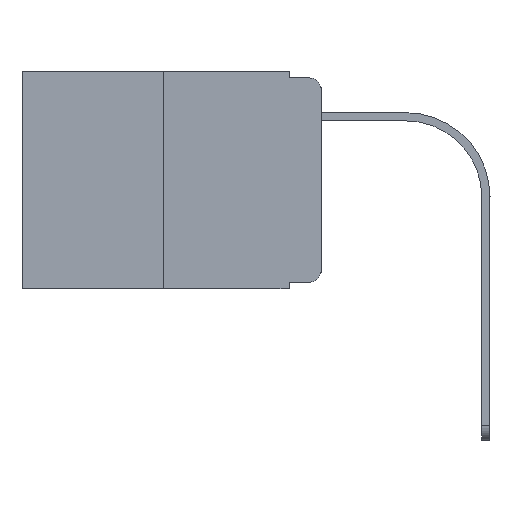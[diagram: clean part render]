
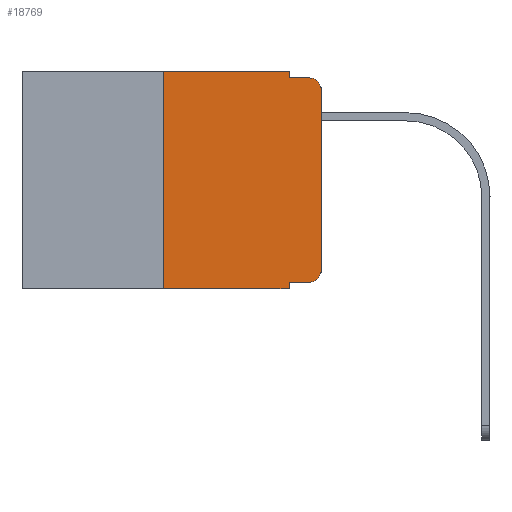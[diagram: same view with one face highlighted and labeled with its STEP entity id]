
A CAD part, left-side view. The second image highlights one B-rep face of the part: STEP entity #18769.
In plain terms, the highlighted planar face has unit normal (-1, 0, 0).
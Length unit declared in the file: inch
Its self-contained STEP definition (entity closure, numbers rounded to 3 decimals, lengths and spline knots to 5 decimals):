
#757 = CARTESIAN_POINT ( 'NONE',  ( 0., 0.051, 0. ) ) ;
#1291 = EDGE_CURVE ( 'NONE', #17932, #7058, #20796, .T. ) ;
#1302 = CARTESIAN_POINT ( 'NONE',  ( 0., 0.02, -0.03 ) ) ;
#1710 = VECTOR ( 'NONE', #16569, 39.37008 ) ;
#1801 = LINE ( 'NONE', #15837, #15571 ) ;
#2091 = LINE ( 'NONE', #12773, #8432 ) ;
#2322 = DIRECTION ( 'NONE',  ( 0., -1., 0. ) ) ;
#2405 = CARTESIAN_POINT ( 'NONE',  ( 0., 0.051, 0. ) ) ;
#2436 = LINE ( 'NONE', #16945, #10281 ) ;
#2755 = VERTEX_POINT ( 'NONE', #18517 ) ;
#2842 = CARTESIAN_POINT ( 'NONE',  ( 0., 0., -0.313 ) ) ;
#3052 = DIRECTION ( 'NONE',  ( 0., 0., -1. ) ) ;
#3207 = DIRECTION ( 'NONE',  ( 0., 0., -1. ) ) ;
#4050 = DIRECTION ( 'NONE',  ( 0., -1., 0. ) ) ;
#4352 = CIRCLE ( 'NONE', #13968, 0.02 ) ;
#4408 = AXIS2_PLACEMENT_3D ( 'NONE', #8864, #19084, #19208 ) ;
#5575 = CARTESIAN_POINT ( 'NONE',  ( 0., 0.051, -0.343 ) ) ;
#5731 = CARTESIAN_POINT ( 'NONE',  ( 0., 0.25, 0. ) ) ;
#5785 = EDGE_CURVE ( 'NONE', #12706, #19299, #18318, .T. ) ;
#6002 = DIRECTION ( 'NONE',  ( 0., 0., 1. ) ) ;
#6439 = VERTEX_POINT ( 'NONE', #5575 ) ;
#6681 = PLANE ( 'NONE',  #4408 ) ;
#7058 = VERTEX_POINT ( 'NONE', #12872 ) ;
#7110 = FACE_OUTER_BOUND ( 'NONE', #17758, .T. ) ;
#7277 = ORIENTED_EDGE ( 'NONE', *, *, #16275, .T. ) ;
#7278 = CARTESIAN_POINT ( 'NONE',  ( 0., 0.473, 0. ) ) ;
#8432 = VECTOR ( 'NONE', #19842, 39.37008 ) ;
#8864 = CARTESIAN_POINT ( 'NONE',  ( 0., 0.473, 0. ) ) ;
#9947 = CARTESIAN_POINT ( 'NONE',  ( 0., 0.02, -0.313 ) ) ;
#10281 = VECTOR ( 'NONE', #2322, 39.37008 ) ;
#10312 = EDGE_CURVE ( 'NONE', #14915, #22020, #2091, .T. ) ;
#10355 = EDGE_CURVE ( 'NONE', #14915, #6439, #2436, .T. ) ;
#10602 = DIRECTION ( 'NONE',  ( 0., 0., -1. ) ) ;
#10775 = ORIENTED_EDGE ( 'NONE', *, *, #10355, .T. ) ;
#11342 = CARTESIAN_POINT ( 'NONE',  ( 0., 0., 0. ) ) ;
#11962 = CARTESIAN_POINT ( 'NONE',  ( 0., 0.051, -0.333 ) ) ;
#11995 = DIRECTION ( 'NONE',  ( 0., -1., 0. ) ) ;
#12545 = EDGE_CURVE ( 'NONE', #17932, #6439, #1801, .T. ) ;
#12706 = VERTEX_POINT ( 'NONE', #757 ) ;
#12773 = CARTESIAN_POINT ( 'NONE',  ( 0., 0.25, 0. ) ) ;
#12872 = CARTESIAN_POINT ( 'NONE',  ( 0., 0.02, -0.333 ) ) ;
#13108 = VERTEX_POINT ( 'NONE', #14766 ) ;
#13968 = AXIS2_PLACEMENT_3D ( 'NONE', #9947, #21066, #3207 ) ;
#14037 = ORIENTED_EDGE ( 'NONE', *, *, #21819, .T. ) ;
#14766 = CARTESIAN_POINT ( 'NONE',  ( 0., 0.02, -0.01 ) ) ;
#14915 = VERTEX_POINT ( 'NONE', #20787 ) ;
#14977 = ORIENTED_EDGE ( 'NONE', *, *, #22851, .F. ) ;
#15316 = ORIENTED_EDGE ( 'NONE', *, *, #21644, .T. ) ;
#15571 = VECTOR ( 'NONE', #10602, 39.37008 ) ;
#15625 = VERTEX_POINT ( 'NONE', #2842 ) ;
#15837 = CARTESIAN_POINT ( 'NONE',  ( 0., 0.051, 0. ) ) ;
#15996 = CARTESIAN_POINT ( 'NONE',  ( 0., 0.051, -0.01 ) ) ;
#16161 = ORIENTED_EDGE ( 'NONE', *, *, #5785, .F. ) ;
#16275 = EDGE_CURVE ( 'NONE', #2755, #13108, #17343, .T. ) ;
#16297 = LINE ( 'NONE', #11342, #19892 ) ;
#16569 = DIRECTION ( 'NONE',  ( 0., 0., -1. ) ) ;
#16658 = ORIENTED_EDGE ( 'NONE', *, *, #10312, .F. ) ;
#16863 = CARTESIAN_POINT ( 'NONE',  ( 0., 0.051, -0.333 ) ) ;
#16945 = CARTESIAN_POINT ( 'NONE',  ( 0., 0.473, -0.343 ) ) ;
#17343 = CIRCLE ( 'NONE', #17709, 0.02 ) ;
#17374 = VECTOR ( 'NONE', #4050, 39.37008 ) ;
#17709 = AXIS2_PLACEMENT_3D ( 'NONE', #1302, #20683, #3052 ) ;
#17758 = EDGE_LOOP ( 'NONE', ( #15316, #7277, #22328, #16161, #14977, #16658, #10775, #22904, #18558, #14037 ) ) ;
#17929 = VECTOR ( 'NONE', #11995, 39.37008 ) ;
#17932 = VERTEX_POINT ( 'NONE', #11962 ) ;
#17958 = EDGE_CURVE ( 'NONE', #19299, #13108, #22823, .T. ) ;
#18318 = LINE ( 'NONE', #2405, #1710 ) ;
#18517 = CARTESIAN_POINT ( 'NONE',  ( 0., 0., -0.03 ) ) ;
#18558 = ORIENTED_EDGE ( 'NONE', *, *, #1291, .T. ) ;
#18769 = ADVANCED_FACE ( 'NONE', ( #7110 ), #6681, .F. ) ;
#19084 = DIRECTION ( 'NONE',  ( 1., 0., 0. ) ) ;
#19208 = DIRECTION ( 'NONE',  ( 0., 0., -1. ) ) ;
#19299 = VERTEX_POINT ( 'NONE', #15996 ) ;
#19362 = DIRECTION ( 'NONE',  ( 0., -1., 0. ) ) ;
#19465 = CARTESIAN_POINT ( 'NONE',  ( 0., 0.051, -0.01 ) ) ;
#19607 = VECTOR ( 'NONE', #19362, 39.37008 ) ;
#19842 = DIRECTION ( 'NONE',  ( 0., 0., 1. ) ) ;
#19892 = VECTOR ( 'NONE', #6002, 39.37008 ) ;
#20683 = DIRECTION ( 'NONE',  ( -1., 0., 0. ) ) ;
#20787 = CARTESIAN_POINT ( 'NONE',  ( 0., 0.25, -0.343 ) ) ;
#20796 = LINE ( 'NONE', #16863, #17929 ) ;
#21066 = DIRECTION ( 'NONE',  ( -1., 0., 0. ) ) ;
#21644 = EDGE_CURVE ( 'NONE', #15625, #2755, #16297, .T. ) ;
#21654 = LINE ( 'NONE', #7278, #17374 ) ;
#21819 = EDGE_CURVE ( 'NONE', #7058, #15625, #4352, .T. ) ;
#22020 = VERTEX_POINT ( 'NONE', #5731 ) ;
#22328 = ORIENTED_EDGE ( 'NONE', *, *, #17958, .F. ) ;
#22823 = LINE ( 'NONE', #19465, #19607 ) ;
#22851 = EDGE_CURVE ( 'NONE', #22020, #12706, #21654, .T. ) ;
#22904 = ORIENTED_EDGE ( 'NONE', *, *, #12545, .F. ) ;
